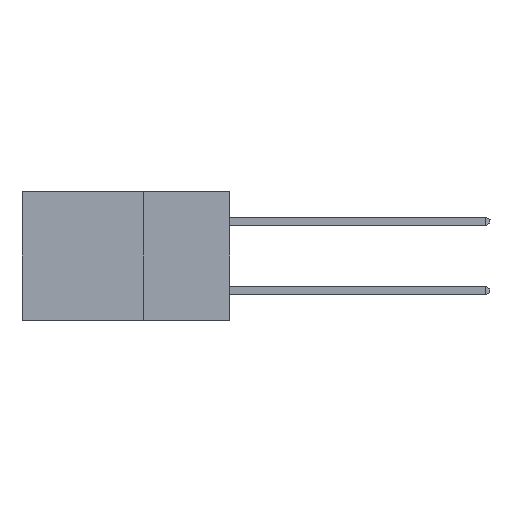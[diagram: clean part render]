
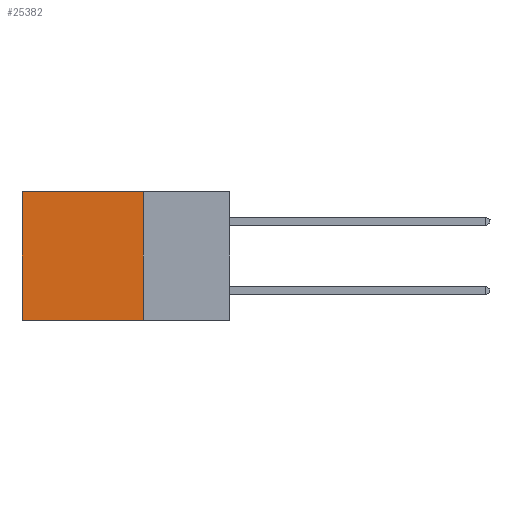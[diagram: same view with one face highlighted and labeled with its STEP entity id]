
A CAD part, left-side view. The second image highlights one B-rep face of the part: STEP entity #25382.
In plain terms, the highlighted planar face has unit normal (-1, 0, 0).
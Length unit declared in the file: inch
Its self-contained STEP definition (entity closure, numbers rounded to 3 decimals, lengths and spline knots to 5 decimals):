
#1380 = AXIS2_PLACEMENT_3D ( 'NONE', #29393, #26905, #21430 ) ;
#2156 = EDGE_CURVE ( 'NONE', #27851, #8645, #2836, .T. ) ;
#2836 = LINE ( 'NONE', #10158, #23956 ) ;
#3439 = ORIENTED_EDGE ( 'NONE', *, *, #7794, .F. ) ;
#5021 = LINE ( 'NONE', #19488, #10348 ) ;
#5657 = CARTESIAN_POINT ( 'NONE',  ( 0.298, 0.6, 0. ) ) ;
#6114 = DIRECTION ( 'NONE',  ( 0., 0., -1. ) ) ;
#7794 = EDGE_CURVE ( 'NONE', #29859, #27851, #15941, .T. ) ;
#8645 = VERTEX_POINT ( 'NONE', #20768 ) ;
#8921 = VECTOR ( 'NONE', #6114, 39.37008 ) ;
#9245 = VERTEX_POINT ( 'NONE', #5657 ) ;
#10158 = CARTESIAN_POINT ( 'NONE',  ( 0.298, 0.25, -0.37 ) ) ;
#10348 = VECTOR ( 'NONE', #27175, 39.37008 ) ;
#10662 = CARTESIAN_POINT ( 'NONE',  ( 0.298, 0.25, 0. ) ) ;
#11604 = DIRECTION ( 'NONE',  ( 0., 1., 0. ) ) ;
#15941 = LINE ( 'NONE', #32563, #8921 ) ;
#16274 = EDGE_CURVE ( 'NONE', #9245, #8645, #5021, .T. ) ;
#17986 = FACE_OUTER_BOUND ( 'NONE', #34038, .T. ) ;
#19488 = CARTESIAN_POINT ( 'NONE',  ( 0.298, 0.6, 0. ) ) ;
#20768 = CARTESIAN_POINT ( 'NONE',  ( 0.298, 0.6, -0.37 ) ) ;
#21075 = CARTESIAN_POINT ( 'NONE',  ( 0.298, 0.25, 0. ) ) ;
#21430 = DIRECTION ( 'NONE',  ( 0., 0., -1. ) ) ;
#23956 = VECTOR ( 'NONE', #11604, 39.37008 ) ;
#24831 = VECTOR ( 'NONE', #29261, 39.37008 ) ;
#25291 = ORIENTED_EDGE ( 'NONE', *, *, #2156, .F. ) ;
#25382 = ADVANCED_FACE ( 'NONE', ( #17986 ), #28909, .F. ) ;
#25512 = CARTESIAN_POINT ( 'NONE',  ( 0.298, 0.25, -0.37 ) ) ;
#26905 = DIRECTION ( 'NONE',  ( 1., 0., 0. ) ) ;
#27175 = DIRECTION ( 'NONE',  ( 0., 0., -1. ) ) ;
#27851 = VERTEX_POINT ( 'NONE', #25512 ) ;
#28827 = EDGE_CURVE ( 'NONE', #29859, #9245, #33217, .T. ) ;
#28909 = PLANE ( 'NONE',  #1380 ) ;
#29261 = DIRECTION ( 'NONE',  ( 0., 1., 0. ) ) ;
#29393 = CARTESIAN_POINT ( 'NONE',  ( 0.298, 0.25, 0. ) ) ;
#29859 = VERTEX_POINT ( 'NONE', #10662 ) ;
#30254 = ORIENTED_EDGE ( 'NONE', *, *, #16274, .T. ) ;
#32104 = ORIENTED_EDGE ( 'NONE', *, *, #28827, .T. ) ;
#32563 = CARTESIAN_POINT ( 'NONE',  ( 0.298, 0.25, 0. ) ) ;
#33217 = LINE ( 'NONE', #21075, #24831 ) ;
#34038 = EDGE_LOOP ( 'NONE', ( #30254, #25291, #3439, #32104 ) ) ;
